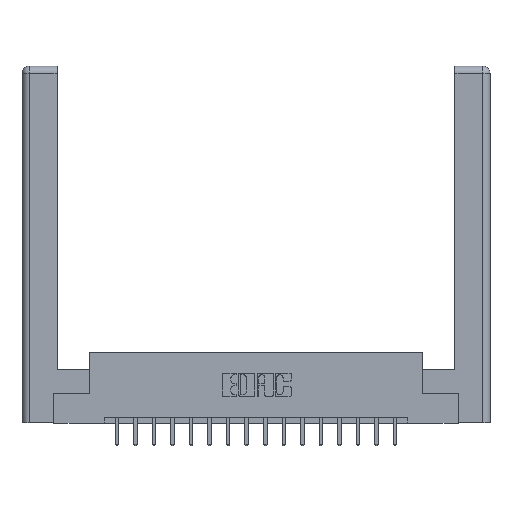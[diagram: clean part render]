
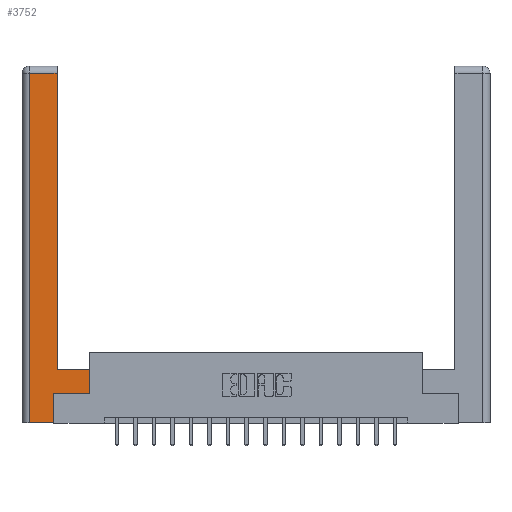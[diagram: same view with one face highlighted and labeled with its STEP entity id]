
A CAD part, top view. The second image highlights one B-rep face of the part: STEP entity #3752.
In plain terms, the highlighted planar face has unit normal (0, 0, 1).
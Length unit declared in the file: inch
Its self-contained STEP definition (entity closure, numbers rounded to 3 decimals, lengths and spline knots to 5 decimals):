
#43 = CARTESIAN_POINT ( 'NONE',  ( 0.295, 0.45, 0. ) ) ;
#251 = EDGE_CURVE ( 'NONE', #10074, #3317, #7950, .T. ) ;
#362 = VECTOR ( 'NONE', #1466, 39.37008 ) ;
#405 = ORIENTED_EDGE ( 'NONE', *, *, #4987, .T. ) ;
#480 = VECTOR ( 'NONE', #6706, 39.37008 ) ;
#1098 = LINE ( 'NONE', #18504, #11383 ) ;
#1142 = LINE ( 'NONE', #9521, #480 ) ;
#1466 = DIRECTION ( 'NONE',  ( 0., 1., 0. ) ) ;
#1610 = CARTESIAN_POINT ( 'NONE',  ( 0.295, 2.94, 0. ) ) ;
#1749 = CARTESIAN_POINT ( 'NONE',  ( 0.0615, 2.94, 0. ) ) ;
#1793 = DIRECTION ( 'NONE',  ( 1., 0., 0. ) ) ;
#1803 = LINE ( 'NONE', #43, #14087 ) ;
#2137 = DIRECTION ( 'NONE',  ( -1., 0., 0. ) ) ;
#2768 = DIRECTION ( 'NONE',  ( 0., -1., 0. ) ) ;
#3317 = VERTEX_POINT ( 'NONE', #1610 ) ;
#3398 = FACE_OUTER_BOUND ( 'NONE', #13691, .T. ) ;
#3752 = ADVANCED_FACE ( 'NONE', ( #3398 ), #11266, .F. ) ;
#3778 = EDGE_CURVE ( 'NONE', #8274, #4089, #12523, .T. ) ;
#3881 = LINE ( 'NONE', #1749, #18452 ) ;
#4089 = VERTEX_POINT ( 'NONE', #18055 ) ;
#4987 = EDGE_CURVE ( 'NONE', #6875, #17425, #11591, .T. ) ;
#5815 = ORIENTED_EDGE ( 'NONE', *, *, #13967, .T. ) ;
#5879 = CARTESIAN_POINT ( 'NONE',  ( 0.565, 0.245, 0. ) ) ;
#5899 = VECTOR ( 'NONE', #7528, 39.37008 ) ;
#6706 = DIRECTION ( 'NONE',  ( 0., 1., 0. ) ) ;
#6753 = VERTEX_POINT ( 'NONE', #16976 ) ;
#6875 = VERTEX_POINT ( 'NONE', #12963 ) ;
#6879 = ORIENTED_EDGE ( 'NONE', *, *, #10969, .T. ) ;
#6991 = DIRECTION ( 'NONE',  ( 0., 1., 0. ) ) ;
#7528 = DIRECTION ( 'NONE',  ( 1., 0., 0. ) ) ;
#7950 = LINE ( 'NONE', #17352, #362 ) ;
#8213 = EDGE_CURVE ( 'NONE', #9608, #8274, #11490, .T. ) ;
#8274 = VERTEX_POINT ( 'NONE', #5879 ) ;
#8578 = CARTESIAN_POINT ( 'NONE',  ( 0.265, 0., 0. ) ) ;
#9024 = CARTESIAN_POINT ( 'NONE',  ( 0.565, 0.245, 0. ) ) ;
#9213 = CARTESIAN_POINT ( 'NONE',  ( 0.295, 0.45, 0. ) ) ;
#9521 = CARTESIAN_POINT ( 'NONE',  ( 0.265, 0.245, 0. ) ) ;
#9608 = VERTEX_POINT ( 'NONE', #15456 ) ;
#9645 = ORIENTED_EDGE ( 'NONE', *, *, #14180, .T. ) ;
#10002 = DIRECTION ( 'NONE',  ( -1., 0., 0. ) ) ;
#10074 = VERTEX_POINT ( 'NONE', #9213 ) ;
#10969 = EDGE_CURVE ( 'NONE', #6753, #6875, #1098, .T. ) ;
#11266 = PLANE ( 'NONE',  #14497 ) ;
#11383 = VECTOR ( 'NONE', #2768, 39.37008 ) ;
#11490 = LINE ( 'NONE', #9024, #5899 ) ;
#11591 = LINE ( 'NONE', #16302, #14267 ) ;
#12146 = ORIENTED_EDGE ( 'NONE', *, *, #8213, .T. ) ;
#12331 = ORIENTED_EDGE ( 'NONE', *, *, #251, .T. ) ;
#12523 = LINE ( 'NONE', #12812, #15012 ) ;
#12812 = CARTESIAN_POINT ( 'NONE',  ( 0.565, 0.45, 0. ) ) ;
#12963 = CARTESIAN_POINT ( 'NONE',  ( 0.0615, 0., 0. ) ) ;
#13001 = DIRECTION ( 'NONE',  ( -1., 0., 0. ) ) ;
#13072 = EDGE_CURVE ( 'NONE', #3317, #6753, #3881, .T. ) ;
#13691 = EDGE_LOOP ( 'NONE', ( #12331, #13948, #6879, #405, #5815, #12146, #13836, #9645 ) ) ;
#13836 = ORIENTED_EDGE ( 'NONE', *, *, #3778, .T. ) ;
#13948 = ORIENTED_EDGE ( 'NONE', *, *, #13072, .T. ) ;
#13967 = EDGE_CURVE ( 'NONE', #17425, #9608, #1142, .T. ) ;
#14087 = VECTOR ( 'NONE', #13001, 39.37008 ) ;
#14180 = EDGE_CURVE ( 'NONE', #4089, #10074, #1803, .T. ) ;
#14267 = VECTOR ( 'NONE', #1793, 39.37008 ) ;
#14497 = AXIS2_PLACEMENT_3D ( 'NONE', #17007, #15653, #10002 ) ;
#15012 = VECTOR ( 'NONE', #6991, 39.37008 ) ;
#15456 = CARTESIAN_POINT ( 'NONE',  ( 0.265, 0.245, 0. ) ) ;
#15653 = DIRECTION ( 'NONE',  ( 0., 0., -1. ) ) ;
#16302 = CARTESIAN_POINT ( 'NONE',  ( 0.265, 0., 0. ) ) ;
#16976 = CARTESIAN_POINT ( 'NONE',  ( 0.0615, 2.94, 0. ) ) ;
#17007 = CARTESIAN_POINT ( 'NONE',  ( 0., 0., 0. ) ) ;
#17352 = CARTESIAN_POINT ( 'NONE',  ( 0.295, 3., 0. ) ) ;
#17425 = VERTEX_POINT ( 'NONE', #8578 ) ;
#18055 = CARTESIAN_POINT ( 'NONE',  ( 0.565, 0.45, 0. ) ) ;
#18452 = VECTOR ( 'NONE', #2137, 39.37008 ) ;
#18504 = CARTESIAN_POINT ( 'NONE',  ( 0.0615, 0., 0. ) ) ;
